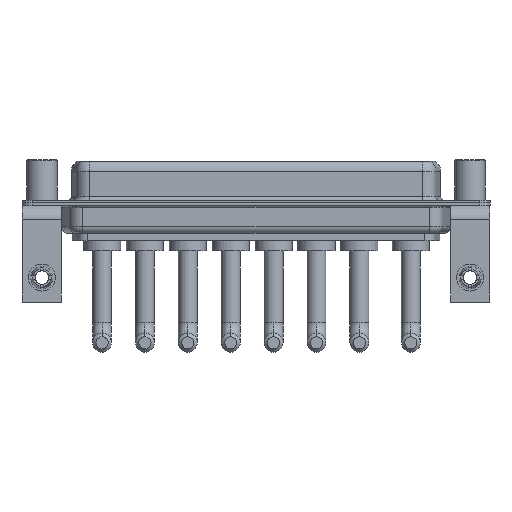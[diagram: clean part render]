
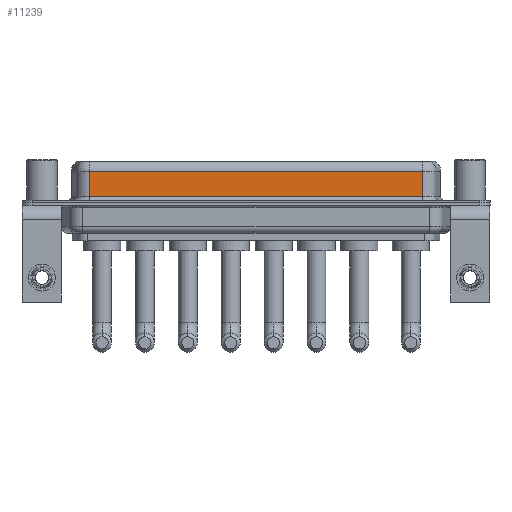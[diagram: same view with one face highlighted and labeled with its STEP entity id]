
A CAD part, front view. The second image highlights one B-rep face of the part: STEP entity #11239.
In plain terms, the highlighted planar face has unit normal (0, -1, 0).
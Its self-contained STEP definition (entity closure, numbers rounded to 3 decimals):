
#101 = CARTESIAN_POINT ( 'NONE',  ( 56.462, -3.95, 6.4 ) ) ;
#830 = DIRECTION ( 'NONE',  ( 1., 0., 0. ) ) ;
#1108 = LINE ( 'NONE', #1195, #5930 ) ;
#1195 = CARTESIAN_POINT ( 'NONE',  ( 7.038, -3.95, 6.4 ) ) ;
#1297 = CARTESIAN_POINT ( 'NONE',  ( 56.462, -3.95, 4.65 ) ) ;
#2165 = DIRECTION ( 'NONE',  ( 0., 1., 0. ) ) ;
#2471 = LINE ( 'NONE', #101, #2883 ) ;
#2555 = DIRECTION ( 'NONE',  ( 0., 0., -1. ) ) ;
#2835 = ORIENTED_EDGE ( 'NONE', *, *, #11689, .T. ) ;
#2883 = VECTOR ( 'NONE', #2555, 1000. ) ;
#4490 = EDGE_CURVE ( 'NONE', #8277, #13472, #15371, .T. ) ;
#5168 = FACE_OUTER_BOUND ( 'NONE', #12813, .T. ) ;
#5930 = VECTOR ( 'NONE', #14750, 1000. ) ;
#5968 = CARTESIAN_POINT ( 'NONE',  ( 7.038, -3.95, 4.65 ) ) ;
#6476 = CARTESIAN_POINT ( 'NONE',  ( 56.462, -3.95, 0.9 ) ) ;
#7320 = VECTOR ( 'NONE', #14131, 1000. ) ;
#8277 = VERTEX_POINT ( 'NONE', #1297 ) ;
#8492 = AXIS2_PLACEMENT_3D ( 'NONE', #10526, #2165, #11842 ) ;
#8921 = EDGE_CURVE ( 'NONE', #13472, #15517, #1108, .T. ) ;
#9335 = VECTOR ( 'NONE', #830, 1000. ) ;
#10526 = CARTESIAN_POINT ( 'NONE',  ( 56.462, -3.95, 6.4 ) ) ;
#10643 = CARTESIAN_POINT ( 'NONE',  ( 56.462, -3.95, 0.9 ) ) ;
#10738 = CARTESIAN_POINT ( 'NONE',  ( 7.038, -3.95, 0.9 ) ) ;
#11065 = ORIENTED_EDGE ( 'NONE', *, *, #8921, .T. ) ;
#11239 = ADVANCED_FACE ( 'NONE', ( #5168 ), #14411, .F. ) ;
#11689 = EDGE_CURVE ( 'NONE', #15517, #13732, #14391, .T. ) ;
#11842 = DIRECTION ( 'NONE',  ( 0., 0., 1. ) ) ;
#12640 = EDGE_CURVE ( 'NONE', #8277, #13732, #2471, .T. ) ;
#12813 = EDGE_LOOP ( 'NONE', ( #16828, #13990, #11065, #2835 ) ) ;
#13472 = VERTEX_POINT ( 'NONE', #5968 ) ;
#13732 = VERTEX_POINT ( 'NONE', #10643 ) ;
#13990 = ORIENTED_EDGE ( 'NONE', *, *, #4490, .T. ) ;
#14131 = DIRECTION ( 'NONE',  ( -1., 0., 0. ) ) ;
#14391 = LINE ( 'NONE', #6476, #9335 ) ;
#14411 = PLANE ( 'NONE',  #8492 ) ;
#14750 = DIRECTION ( 'NONE',  ( 0., 0., -1. ) ) ;
#15371 = LINE ( 'NONE', #15555, #7320 ) ;
#15517 = VERTEX_POINT ( 'NONE', #10738 ) ;
#15555 = CARTESIAN_POINT ( 'NONE',  ( 56.462, -3.95, 4.65 ) ) ;
#16828 = ORIENTED_EDGE ( 'NONE', *, *, #12640, .F. ) ;
